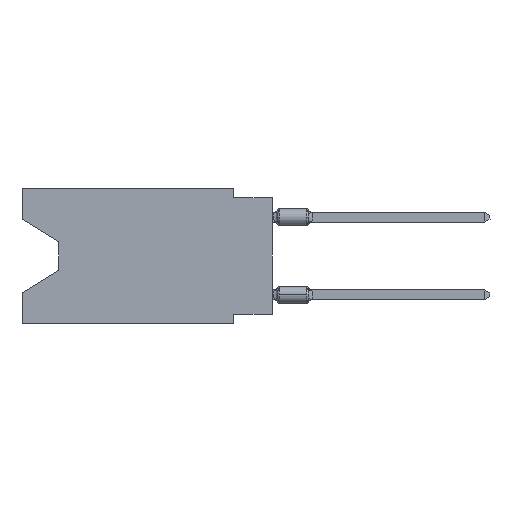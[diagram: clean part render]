
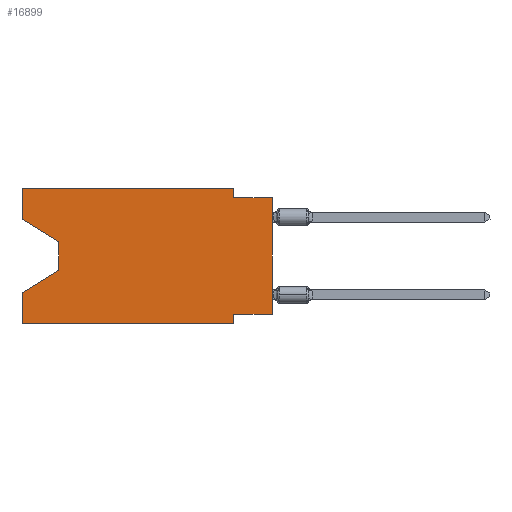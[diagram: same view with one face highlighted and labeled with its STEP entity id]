
A CAD part, left-side view. The second image highlights one B-rep face of the part: STEP entity #16899.
In plain terms, the highlighted planar face has unit normal (-1, 0, 0).
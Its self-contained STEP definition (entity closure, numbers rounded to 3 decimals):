
#46 = ORIENTED_EDGE ( 'NONE', *, *, #19228, .T. ) ;
#68 = LINE ( 'NONE', #17790, #9907 ) ;
#226 = FACE_OUTER_BOUND ( 'NONE', #20388, .T. ) ;
#649 = DIRECTION ( 'NONE',  ( 0., 1., 0. ) ) ;
#766 = EDGE_CURVE ( 'NONE', #9045, #16168, #10697, .T. ) ;
#783 = ORIENTED_EDGE ( 'NONE', *, *, #10085, .F. ) ;
#829 = CARTESIAN_POINT ( 'NONE',  ( 0., 2.54, -8.255 ) ) ;
#1047 = VERTEX_POINT ( 'NONE', #19386 ) ;
#1176 = LINE ( 'NONE', #4182, #6749 ) ;
#1241 = EDGE_CURVE ( 'NONE', #5917, #11393, #7237, .T. ) ;
#1247 = DIRECTION ( 'NONE',  ( 0., 0., -1. ) ) ;
#1273 = DIRECTION ( 'NONE',  ( 0., 0., 1. ) ) ;
#1470 = DIRECTION ( 'NONE',  ( 0., -1., 0. ) ) ;
#2179 = EDGE_CURVE ( 'NONE', #2799, #9045, #4469, .T. ) ;
#2228 = ORIENTED_EDGE ( 'NONE', *, *, #2991, .F. ) ;
#2338 = VECTOR ( 'NONE', #17979, 1000. ) ;
#2525 = CARTESIAN_POINT ( 'NONE',  ( 0., 16.383, 0. ) ) ;
#2561 = CARTESIAN_POINT ( 'NONE',  ( 0., 0., -8.255 ) ) ;
#2799 = VERTEX_POINT ( 'NONE', #6580 ) ;
#2991 = EDGE_CURVE ( 'NONE', #2799, #12075, #3890, .T. ) ;
#3223 = PLANE ( 'NONE',  #6638 ) ;
#3304 = VERTEX_POINT ( 'NONE', #15039 ) ;
#3346 = CARTESIAN_POINT ( 'NONE',  ( 0., 16.383, 0. ) ) ;
#3890 = LINE ( 'NONE', #18183, #3977 ) ;
#3977 = VECTOR ( 'NONE', #10435, 1000. ) ;
#4003 = DIRECTION ( 'NONE',  ( 0., 0., -1. ) ) ;
#4151 = CARTESIAN_POINT ( 'NONE',  ( 0., 16.383, -2.038 ) ) ;
#4182 = CARTESIAN_POINT ( 'NONE',  ( 0., 0., -0.635 ) ) ;
#4239 = EDGE_CURVE ( 'NONE', #17305, #19496, #8608, .T. ) ;
#4356 = VECTOR ( 'NONE', #4003, 1000. ) ;
#4469 = LINE ( 'NONE', #4151, #5324 ) ;
#4671 = LINE ( 'NONE', #19380, #8458 ) ;
#4838 = DIRECTION ( 'NONE',  ( 0., 0., -1. ) ) ;
#5324 = VECTOR ( 'NONE', #5968, 1000. ) ;
#5709 = VECTOR ( 'NONE', #649, 1000. ) ;
#5917 = VERTEX_POINT ( 'NONE', #11941 ) ;
#5968 = DIRECTION ( 'NONE',  ( 0., -0.855, -0.519 ) ) ;
#6402 = CARTESIAN_POINT ( 'NONE',  ( 0., 16.383, -8.89 ) ) ;
#6580 = CARTESIAN_POINT ( 'NONE',  ( 0., 16.383, -2.038 ) ) ;
#6638 = AXIS2_PLACEMENT_3D ( 'NONE', #3346, #9770, #4838 ) ;
#6749 = VECTOR ( 'NONE', #15772, 1000. ) ;
#6913 = LINE ( 'NONE', #10868, #14185 ) ;
#7180 = EDGE_CURVE ( 'NONE', #16168, #11393, #6913, .T. ) ;
#7237 = LINE ( 'NONE', #2525, #7362 ) ;
#7362 = VECTOR ( 'NONE', #15720, 1000. ) ;
#8000 = EDGE_CURVE ( 'NONE', #1047, #17305, #15643, .T. ) ;
#8424 = ORIENTED_EDGE ( 'NONE', *, *, #8000, .F. ) ;
#8458 = VECTOR ( 'NONE', #1247, 1000. ) ;
#8608 = LINE ( 'NONE', #18397, #4356 ) ;
#8777 = CARTESIAN_POINT ( 'NONE',  ( 0., 13.97, -3.505 ) ) ;
#8971 = CARTESIAN_POINT ( 'NONE',  ( 0., 13.97, -3.505 ) ) ;
#9045 = VERTEX_POINT ( 'NONE', #8777 ) ;
#9288 = EDGE_CURVE ( 'NONE', #1047, #16810, #15954, .T. ) ;
#9611 = ORIENTED_EDGE ( 'NONE', *, *, #11788, .F. ) ;
#9770 = DIRECTION ( 'NONE',  ( 1., 0., 0. ) ) ;
#9907 = VECTOR ( 'NONE', #1470, 1000. ) ;
#10047 = ORIENTED_EDGE ( 'NONE', *, *, #9288, .T. ) ;
#10085 = EDGE_CURVE ( 'NONE', #15516, #16810, #1176, .T. ) ;
#10435 = DIRECTION ( 'NONE',  ( 0., 0., 1. ) ) ;
#10697 = LINE ( 'NONE', #8971, #21093 ) ;
#10868 = CARTESIAN_POINT ( 'NONE',  ( 0., 13.97, -5.385 ) ) ;
#11339 = ORIENTED_EDGE ( 'NONE', *, *, #766, .T. ) ;
#11393 = VERTEX_POINT ( 'NONE', #19745 ) ;
#11788 = EDGE_CURVE ( 'NONE', #12075, #3304, #68, .T. ) ;
#11941 = CARTESIAN_POINT ( 'NONE',  ( 0., 16.383, -8.89 ) ) ;
#12075 = VERTEX_POINT ( 'NONE', #20681 ) ;
#14101 = CARTESIAN_POINT ( 'NONE',  ( 0., 2.54, -8.89 ) ) ;
#14167 = CARTESIAN_POINT ( 'NONE',  ( 0., 2.54, -0.635 ) ) ;
#14185 = VECTOR ( 'NONE', #18832, 1000. ) ;
#14697 = EDGE_CURVE ( 'NONE', #3304, #15516, #4671, .T. ) ;
#14773 = ORIENTED_EDGE ( 'NONE', *, *, #14697, .F. ) ;
#15039 = CARTESIAN_POINT ( 'NONE',  ( 0., 2.54, 0. ) ) ;
#15516 = VERTEX_POINT ( 'NONE', #14167 ) ;
#15528 = DIRECTION ( 'NONE',  ( 0., 0., -1. ) ) ;
#15643 = LINE ( 'NONE', #2561, #5709 ) ;
#15720 = DIRECTION ( 'NONE',  ( 0., 0., 1. ) ) ;
#15772 = DIRECTION ( 'NONE',  ( 0., -1., 0. ) ) ;
#15954 = LINE ( 'NONE', #17573, #20125 ) ;
#16168 = VERTEX_POINT ( 'NONE', #20281 ) ;
#16203 = CARTESIAN_POINT ( 'NONE',  ( 0., 0., -0.635 ) ) ;
#16810 = VERTEX_POINT ( 'NONE', #16203 ) ;
#16899 = ADVANCED_FACE ( 'NONE', ( #226 ), #3223, .F. ) ;
#17305 = VERTEX_POINT ( 'NONE', #829 ) ;
#17399 = ORIENTED_EDGE ( 'NONE', *, *, #1241, .F. ) ;
#17573 = CARTESIAN_POINT ( 'NONE',  ( 0., 0., 0. ) ) ;
#17659 = LINE ( 'NONE', #6402, #2338 ) ;
#17790 = CARTESIAN_POINT ( 'NONE',  ( 0., 16.383, 0. ) ) ;
#17979 = DIRECTION ( 'NONE',  ( 0., -1., 0. ) ) ;
#18183 = CARTESIAN_POINT ( 'NONE',  ( 0., 16.383, 0. ) ) ;
#18397 = CARTESIAN_POINT ( 'NONE',  ( 0., 2.54, -8.89 ) ) ;
#18471 = ORIENTED_EDGE ( 'NONE', *, *, #4239, .F. ) ;
#18479 = ORIENTED_EDGE ( 'NONE', *, *, #2179, .T. ) ;
#18832 = DIRECTION ( 'NONE',  ( 0., 0.855, -0.519 ) ) ;
#19021 = ORIENTED_EDGE ( 'NONE', *, *, #7180, .T. ) ;
#19228 = EDGE_CURVE ( 'NONE', #5917, #19496, #17659, .T. ) ;
#19380 = CARTESIAN_POINT ( 'NONE',  ( 0., 2.54, 0. ) ) ;
#19386 = CARTESIAN_POINT ( 'NONE',  ( 0., 0., -8.255 ) ) ;
#19496 = VERTEX_POINT ( 'NONE', #14101 ) ;
#19745 = CARTESIAN_POINT ( 'NONE',  ( 0., 16.383, -6.852 ) ) ;
#20125 = VECTOR ( 'NONE', #1273, 1000. ) ;
#20281 = CARTESIAN_POINT ( 'NONE',  ( 0., 13.97, -5.385 ) ) ;
#20388 = EDGE_LOOP ( 'NONE', ( #18479, #11339, #19021, #17399, #46, #18471, #8424, #10047, #783, #14773, #9611, #2228 ) ) ;
#20681 = CARTESIAN_POINT ( 'NONE',  ( 0., 16.383, 0. ) ) ;
#21093 = VECTOR ( 'NONE', #15528, 1000. ) ;
